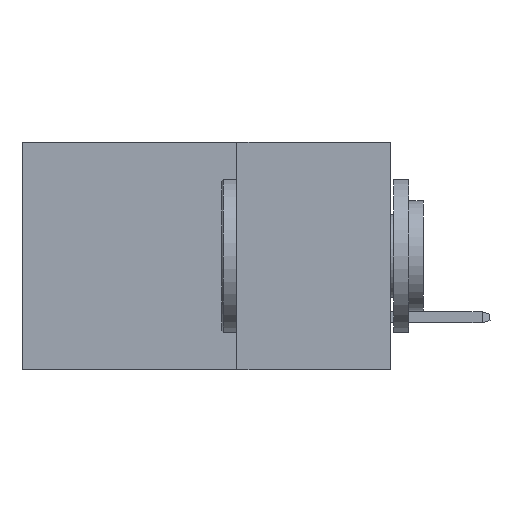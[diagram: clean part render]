
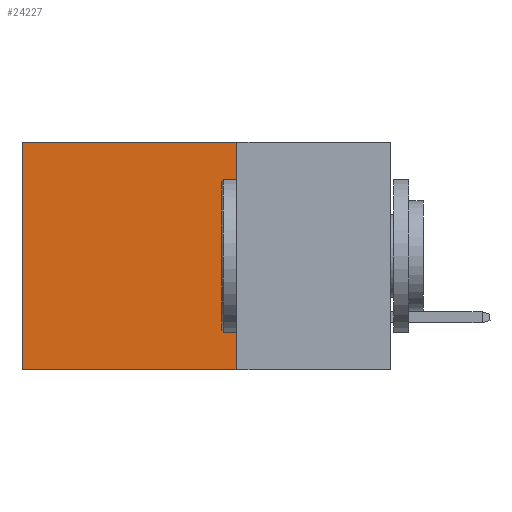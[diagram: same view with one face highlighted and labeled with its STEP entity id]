
A CAD part, left-side view. The second image highlights one B-rep face of the part: STEP entity #24227.
In plain terms, the highlighted planar face has unit normal (-1, 0, 0).
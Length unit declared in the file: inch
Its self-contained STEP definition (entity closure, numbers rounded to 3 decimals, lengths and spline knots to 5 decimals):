
#2229 = CARTESIAN_POINT ( 'NONE',  ( 0.2875, 0.6, 0. ) ) ;
#2303 = CARTESIAN_POINT ( 'NONE',  ( 0.2875, 0.25, 0. ) ) ;
#2447 = ORIENTED_EDGE ( 'NONE', *, *, #5282, .F. ) ;
#2531 = CARTESIAN_POINT ( 'NONE',  ( 0.2875, 0.25, -0.37 ) ) ;
#2596 = EDGE_CURVE ( 'NONE', #17488, #15643, #28427, .T. ) ;
#3334 = FACE_OUTER_BOUND ( 'NONE', #23205, .T. ) ;
#3631 = CARTESIAN_POINT ( 'NONE',  ( 0.2875, 0.6, -0.37 ) ) ;
#5282 = EDGE_CURVE ( 'NONE', #26211, #15643, #19949, .T. ) ;
#6276 = CARTESIAN_POINT ( 'NONE',  ( 0.2875, 0.25, 0. ) ) ;
#8240 = DIRECTION ( 'NONE',  ( 0., 1., 0. ) ) ;
#9861 = DIRECTION ( 'NONE',  ( 0., 0., -1. ) ) ;
#10635 = DIRECTION ( 'NONE',  ( 1., 0., 0. ) ) ;
#10665 = CARTESIAN_POINT ( 'NONE',  ( 0.2875, 0.25, -0.37 ) ) ;
#10725 = EDGE_CURVE ( 'NONE', #18287, #26211, #27806, .T. ) ;
#12103 = EDGE_CURVE ( 'NONE', #18287, #17488, #27713, .T. ) ;
#12633 = ORIENTED_EDGE ( 'NONE', *, *, #2596, .T. ) ;
#14104 = VECTOR ( 'NONE', #9861, 39.37008 ) ;
#15643 = VERTEX_POINT ( 'NONE', #3631 ) ;
#17488 = VERTEX_POINT ( 'NONE', #20742 ) ;
#18287 = VERTEX_POINT ( 'NONE', #6276 ) ;
#18369 = CARTESIAN_POINT ( 'NONE',  ( 0.2875, 0.25, 0. ) ) ;
#18520 = DIRECTION ( 'NONE',  ( 0., 1., 0. ) ) ;
#19949 = LINE ( 'NONE', #2531, #32515 ) ;
#20449 = ORIENTED_EDGE ( 'NONE', *, *, #10725, .F. ) ;
#20742 = CARTESIAN_POINT ( 'NONE',  ( 0.2875, 0.6, 0. ) ) ;
#21100 = VECTOR ( 'NONE', #27839, 39.37008 ) ;
#21263 = ORIENTED_EDGE ( 'NONE', *, *, #12103, .T. ) ;
#23159 = AXIS2_PLACEMENT_3D ( 'NONE', #28324, #10635, #28441 ) ;
#23205 = EDGE_LOOP ( 'NONE', ( #12633, #2447, #20449, #21263 ) ) ;
#24227 = ADVANCED_FACE ( 'NONE', ( #3334 ), #25922, .F. ) ;
#25922 = PLANE ( 'NONE',  #23159 ) ;
#26138 = VECTOR ( 'NONE', #8240, 39.37008 ) ;
#26211 = VERTEX_POINT ( 'NONE', #10665 ) ;
#27713 = LINE ( 'NONE', #18369, #26138 ) ;
#27806 = LINE ( 'NONE', #2303, #21100 ) ;
#27839 = DIRECTION ( 'NONE',  ( 0., 0., -1. ) ) ;
#28324 = CARTESIAN_POINT ( 'NONE',  ( 0.2875, 0.25, 0. ) ) ;
#28427 = LINE ( 'NONE', #2229, #14104 ) ;
#28441 = DIRECTION ( 'NONE',  ( 0., 0., -1. ) ) ;
#32515 = VECTOR ( 'NONE', #18520, 39.37008 ) ;
